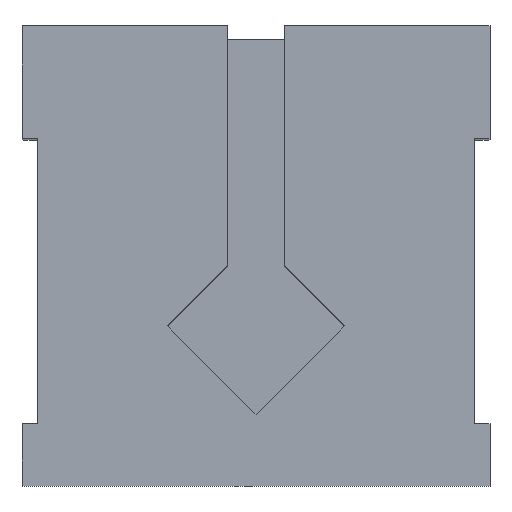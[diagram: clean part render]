
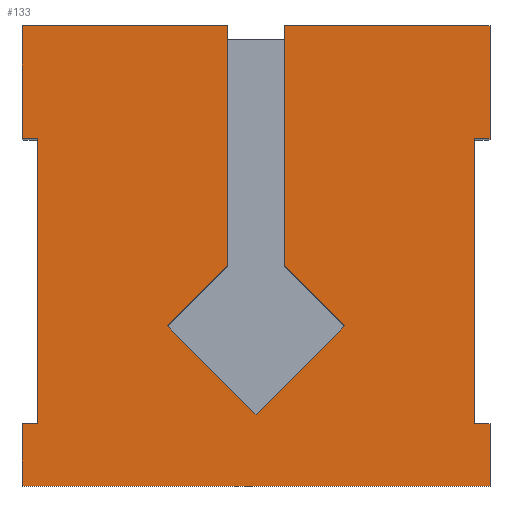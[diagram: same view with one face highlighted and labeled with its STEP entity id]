
A CAD part, top view. The second image highlights one B-rep face of the part: STEP entity #133.
In plain terms, the highlighted planar face has unit normal (0, 0, 1).
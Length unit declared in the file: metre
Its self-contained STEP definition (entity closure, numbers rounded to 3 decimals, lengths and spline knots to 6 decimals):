
#133 = ADVANCED_FACE( '', ( #314 ), #315, .T. );
#314 = FACE_OUTER_BOUND( '', #544, .T. );
#315 = PLANE( '', #545 );
#544 = EDGE_LOOP( '', ( #869, #870, #871, #872, #873, #874, #875, #876, #877, #878, #879, #880, #881, #882, #883, #884, #885, #886, #887 ) );
#545 = AXIS2_PLACEMENT_3D( '', #888, #889, #890 );
#869 = ORIENTED_EDGE( '', *, *, #1490, .F. );
#870 = ORIENTED_EDGE( '', *, *, #1553, .F. );
#871 = ORIENTED_EDGE( '', *, *, #1548, .F. );
#872 = ORIENTED_EDGE( '', *, *, #1554, .T. );
#873 = ORIENTED_EDGE( '', *, *, #1485, .T. );
#874 = ORIENTED_EDGE( '', *, *, #1555, .F. );
#875 = ORIENTED_EDGE( '', *, *, #1556, .F. );
#876 = ORIENTED_EDGE( '', *, *, #1557, .T. );
#877 = ORIENTED_EDGE( '', *, *, #1558, .T. );
#878 = ORIENTED_EDGE( '', *, *, #1559, .T. );
#879 = ORIENTED_EDGE( '', *, *, #1560, .F. );
#880 = ORIENTED_EDGE( '', *, *, #1561, .F. );
#881 = ORIENTED_EDGE( '', *, *, #1562, .T. );
#882 = ORIENTED_EDGE( '', *, *, #1563, .F. );
#883 = ORIENTED_EDGE( '', *, *, #1564, .T. );
#884 = ORIENTED_EDGE( '', *, *, #1565, .F. );
#885 = ORIENTED_EDGE( '', *, *, #1566, .F. );
#886 = ORIENTED_EDGE( '', *, *, #1567, .F. );
#887 = ORIENTED_EDGE( '', *, *, #1568, .F. );
#888 = CARTESIAN_POINT( '', ( 0.022407, 0.02205, 0.02625 ) );
#889 = DIRECTION( '', ( 0., 0., 1. ) );
#890 = DIRECTION( '', ( 1., 0., 0. ) );
#1485 = EDGE_CURVE( '', #1807, #1805, #1808, .T. );
#1490 = EDGE_CURVE( '', #1813, #1816, #1817, .T. );
#1548 = EDGE_CURVE( '', #1917, #1918, #1919, .T. );
#1553 = EDGE_CURVE( '', #1918, #1813, #1926, .T. );
#1554 = EDGE_CURVE( '', #1917, #1807, #1927, .T. );
#1555 = EDGE_CURVE( '', #1928, #1805, #1929, .T. );
#1556 = EDGE_CURVE( '', #1930, #1928, #1931, .T. );
#1557 = EDGE_CURVE( '', #1930, #1932, #1933, .T. );
#1558 = EDGE_CURVE( '', #1932, #1934, #1935, .T. );
#1559 = EDGE_CURVE( '', #1934, #1936, #1937, .T. );
#1560 = EDGE_CURVE( '', #1938, #1936, #1939, .T. );
#1561 = EDGE_CURVE( '', #1940, #1938, #1941, .T. );
#1562 = EDGE_CURVE( '', #1940, #1942, #1943, .T. );
#1563 = EDGE_CURVE( '', #1944, #1942, #1945, .T. );
#1564 = EDGE_CURVE( '', #1944, #1946, #1947, .T. );
#1565 = EDGE_CURVE( '', #1948, #1946, #1949, .T. );
#1566 = EDGE_CURVE( '', #1950, #1948, #1951, .T. );
#1567 = EDGE_CURVE( '', #1952, #1950, #1953, .T. );
#1568 = EDGE_CURVE( '', #1816, #1952, #1954, .T. );
#1805 = VERTEX_POINT( '', #2269 );
#1807 = VERTEX_POINT( '', #2272 );
#1808 = LINE( '', #2273, #2274 );
#1813 = VERTEX_POINT( '', #2280 );
#1816 = VERTEX_POINT( '', #2284 );
#1817 = LINE( '', #2285, #2286 );
#1917 = VERTEX_POINT( '', #2420 );
#1918 = VERTEX_POINT( '', #2421 );
#1919 = LINE( '', #2422, #2423 );
#1926 = LINE( '', #2433, #2434 );
#1927 = LINE( '', #2435, #2436 );
#1928 = VERTEX_POINT( '', #2437 );
#1929 = LINE( '', #2438, #2439 );
#1930 = VERTEX_POINT( '', #2440 );
#1931 = LINE( '', #2441, #2442 );
#1932 = VERTEX_POINT( '', #2443 );
#1933 = LINE( '', #2444, #2445 );
#1934 = VERTEX_POINT( '', #2446 );
#1935 = LINE( '', #2447, #2448 );
#1936 = VERTEX_POINT( '', #2449 );
#1937 = LINE( '', #2450, #2451 );
#1938 = VERTEX_POINT( '', #2452 );
#1939 = LINE( '', #2453, #2454 );
#1940 = VERTEX_POINT( '', #2455 );
#1941 = LINE( '', #2456, #2457 );
#1942 = VERTEX_POINT( '', #2458 );
#1943 = LINE( '', #2459, #2460 );
#1944 = VERTEX_POINT( '', #2461 );
#1945 = LINE( '', #2462, #2463 );
#1946 = VERTEX_POINT( '', #2464 );
#1947 = LINE( '', #2465, #2466 );
#1948 = VERTEX_POINT( '', #2467 );
#1949 = LINE( '', #2468, #2469 );
#1950 = VERTEX_POINT( '', #2470 );
#1951 = LINE( '', #2471, #2472 );
#1952 = VERTEX_POINT( '', #2473 );
#1953 = LINE( '', #2474, #2475 );
#1954 = LINE( '', #2476, #2477 );
#2269 = CARTESIAN_POINT( '', ( 0.0015, 0.006, 0.02625 ) );
#2272 = CARTESIAN_POINT( '', ( 0.0015, 0.0333, 0.02625 ) );
#2273 = CARTESIAN_POINT( '', ( 0.0015, 0.01965, 0.02625 ) );
#2274 = VECTOR( '', #2868, 1. );
#2280 = CARTESIAN_POINT( '', ( 0.019657, 0.0441, 0.02625 ) );
#2284 = CARTESIAN_POINT( '', ( 0.019657, 0.0211, 0.02625 ) );
#2285 = CARTESIAN_POINT( '', ( 0.019657, 0.0326, 0.02625 ) );
#2286 = VECTOR( '', #2874, 1. );
#2420 = CARTESIAN_POINT( '', ( 0., 0.0333, 0.02625 ) );
#2421 = CARTESIAN_POINT( '', ( 0., 0.0441, 0.02625 ) );
#2422 = CARTESIAN_POINT( '', ( 0., 0.0387, 0.02625 ) );
#2423 = VECTOR( '', #2945, 1. );
#2433 = CARTESIAN_POINT( '', ( 0.009829, 0.0441, 0.02625 ) );
#2434 = VECTOR( '', #2949, 1. );
#2435 = CARTESIAN_POINT( '', ( 0.00075, 0.0333, 0.02625 ) );
#2436 = VECTOR( '', #2950, 1. );
#2437 = CARTESIAN_POINT( '', ( 0., 0.006, 0.02625 ) );
#2438 = CARTESIAN_POINT( '', ( 0.00075, 0.006, 0.02625 ) );
#2439 = VECTOR( '', #2951, 1. );
#2440 = CARTESIAN_POINT( '', ( 0., 0., 0.02625 ) );
#2441 = CARTESIAN_POINT( '', ( 0., 0.003, 0.02625 ) );
#2442 = VECTOR( '', #2952, 1. );
#2443 = CARTESIAN_POINT( '', ( 0.044814, 0., 0.02625 ) );
#2444 = CARTESIAN_POINT( '', ( 0.022407, 0., 0.02625 ) );
#2445 = VECTOR( '', #2953, 1. );
#2446 = CARTESIAN_POINT( '', ( 0.044814, 0.006, 0.02625 ) );
#2447 = CARTESIAN_POINT( '', ( 0.044814, 0.003, 0.02625 ) );
#2448 = VECTOR( '', #2954, 1. );
#2449 = CARTESIAN_POINT( '', ( 0.043314, 0.006, 0.02625 ) );
#2450 = CARTESIAN_POINT( '', ( 0.044064, 0.006, 0.02625 ) );
#2451 = VECTOR( '', #2955, 1. );
#2452 = CARTESIAN_POINT( '', ( 0.043314, 0.0333, 0.02625 ) );
#2453 = CARTESIAN_POINT( '', ( 0.043314, 0.01965, 0.02625 ) );
#2454 = VECTOR( '', #2956, 1. );
#2455 = CARTESIAN_POINT( '', ( 0.044814, 0.0333, 0.02625 ) );
#2456 = CARTESIAN_POINT( '', ( 0.044064, 0.0333, 0.02625 ) );
#2457 = VECTOR( '', #2957, 1. );
#2458 = CARTESIAN_POINT( '', ( 0.044814, 0.0441, 0.02625 ) );
#2459 = CARTESIAN_POINT( '', ( 0.044814, 0.0387, 0.02625 ) );
#2460 = VECTOR( '', #2958, 1. );
#2461 = CARTESIAN_POINT( '', ( 0.025157, 0.0441, 0.02625 ) );
#2462 = CARTESIAN_POINT( '', ( 0.034986, 0.0441, 0.02625 ) );
#2463 = VECTOR( '', #2959, 1. );
#2464 = CARTESIAN_POINT( '', ( 0.025157, 0.0211, 0.02625 ) );
#2465 = CARTESIAN_POINT( '', ( 0.025157, 0.0326, 0.02625 ) );
#2466 = VECTOR( '', #2960, 1. );
#2467 = CARTESIAN_POINT( '', ( 0.030907, 0.01535, 0.02625 ) );
#2468 = CARTESIAN_POINT( '', ( 0.028032, 0.018225, 0.02625 ) );
#2469 = VECTOR( '', #2961, 1. );
#2470 = CARTESIAN_POINT( '', ( 0.022407, 0.00685, 0.02625 ) );
#2471 = CARTESIAN_POINT( '', ( 0.026657, 0.0111, 0.02625 ) );
#2472 = VECTOR( '', #2962, 1. );
#2473 = CARTESIAN_POINT( '', ( 0.013907, 0.01535, 0.02625 ) );
#2474 = CARTESIAN_POINT( '', ( 0.018157, 0.0111, 0.02625 ) );
#2475 = VECTOR( '', #2963, 1. );
#2476 = CARTESIAN_POINT( '', ( 0.016782, 0.018225, 0.02625 ) );
#2477 = VECTOR( '', #2964, 1. );
#2868 = DIRECTION( '', ( 0., -1., 0. ) );
#2874 = DIRECTION( '', ( 0., -1., 0. ) );
#2945 = DIRECTION( '', ( 0., 1., 0. ) );
#2949 = DIRECTION( '', ( 1., 0., 0. ) );
#2950 = DIRECTION( '', ( 1., 0., 0. ) );
#2951 = DIRECTION( '', ( 1., 0., 0. ) );
#2952 = DIRECTION( '', ( 0., 1., 0. ) );
#2953 = DIRECTION( '', ( 1., 0., 0. ) );
#2954 = DIRECTION( '', ( 0., 1., 0. ) );
#2955 = DIRECTION( '', ( -1., 0., 0. ) );
#2956 = DIRECTION( '', ( 0., -1., 0. ) );
#2957 = DIRECTION( '', ( -1., 0., 0. ) );
#2958 = DIRECTION( '', ( 0., 1., 0. ) );
#2959 = DIRECTION( '', ( 1., 0., 0. ) );
#2960 = DIRECTION( '', ( 0., -1., 0. ) );
#2961 = DIRECTION( '', ( -0.707, 0.707, 0. ) );
#2962 = DIRECTION( '', ( 0.707, 0.707, 0. ) );
#2963 = DIRECTION( '', ( 0.707, -0.707, 0. ) );
#2964 = DIRECTION( '', ( -0.707, -0.707, 0. ) );
